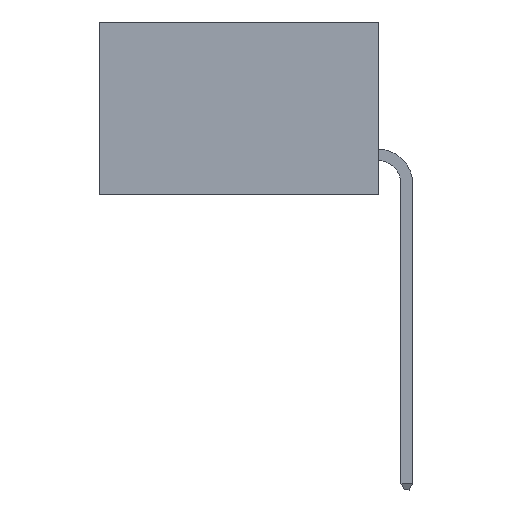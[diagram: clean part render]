
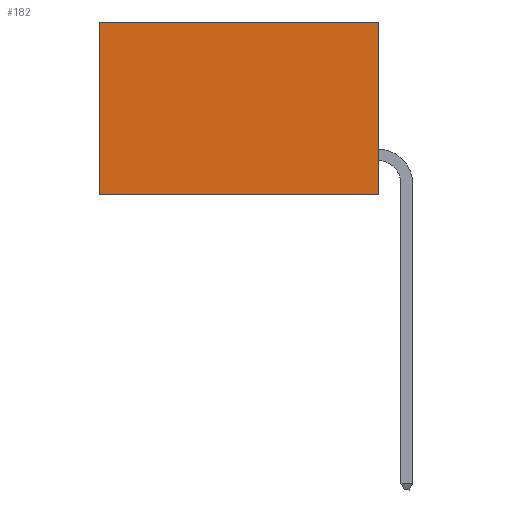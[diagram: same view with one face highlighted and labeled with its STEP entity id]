
A CAD part, left-side view. The second image highlights one B-rep face of the part: STEP entity #182.
In plain terms, the highlighted planar face has unit normal (-1, 0, 0).
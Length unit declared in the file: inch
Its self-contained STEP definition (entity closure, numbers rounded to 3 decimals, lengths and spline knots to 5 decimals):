
#182 = ADVANCED_FACE ( 'NONE', ( #12329 ), #8001, .F. ) ;
#435 = VERTEX_POINT ( 'NONE', #6025 ) ;
#619 = ORIENTED_EDGE ( 'NONE', *, *, #21745, .F. ) ;
#681 = CARTESIAN_POINT ( 'NONE',  ( 0.298, 0., 0. ) ) ;
#2143 = EDGE_LOOP ( 'NONE', ( #9115, #619, #16724, #24660 ) ) ;
#2857 = CARTESIAN_POINT ( 'NONE',  ( 0.298, 0.6, 0. ) ) ;
#3117 = EDGE_CURVE ( 'NONE', #23416, #435, #4865, .T. ) ;
#4064 = DIRECTION ( 'NONE',  ( 0., 1., 0. ) ) ;
#4679 = DIRECTION ( 'NONE',  ( 0., 0., -1. ) ) ;
#4865 = LINE ( 'NONE', #19541, #24991 ) ;
#5903 = LINE ( 'NONE', #12086, #15820 ) ;
#6025 = CARTESIAN_POINT ( 'NONE',  ( 0.298, 0., -0.37 ) ) ;
#6329 = CARTESIAN_POINT ( 'NONE',  ( 0.298, 0.6, -0.37 ) ) ;
#7411 = CARTESIAN_POINT ( 'NONE',  ( 0.298, 0., -0.37 ) ) ;
#7842 = DIRECTION ( 'NONE',  ( 0., 0., -1. ) ) ;
#8001 = PLANE ( 'NONE',  #11946 ) ;
#8317 = DIRECTION ( 'NONE',  ( 1., 0., 0. ) ) ;
#9115 = ORIENTED_EDGE ( 'NONE', *, *, #25028, .T. ) ;
#9404 = DIRECTION ( 'NONE',  ( 0., 1., 0. ) ) ;
#9970 = VERTEX_POINT ( 'NONE', #6329 ) ;
#10816 = VECTOR ( 'NONE', #18681, 39.37008 ) ;
#11425 = LINE ( 'NONE', #2857, #10816 ) ;
#11875 = LINE ( 'NONE', #7411, #21538 ) ;
#11946 = AXIS2_PLACEMENT_3D ( 'NONE', #18312, #8317, #4679 ) ;
#12086 = CARTESIAN_POINT ( 'NONE',  ( 0.298, 0., 0. ) ) ;
#12329 = FACE_OUTER_BOUND ( 'NONE', #2143, .T. ) ;
#15820 = VECTOR ( 'NONE', #4064, 39.37008 ) ;
#16724 = ORIENTED_EDGE ( 'NONE', *, *, #3117, .F. ) ;
#18312 = CARTESIAN_POINT ( 'NONE',  ( 0.298, 0., 0. ) ) ;
#18681 = DIRECTION ( 'NONE',  ( 0., 0., -1. ) ) ;
#19541 = CARTESIAN_POINT ( 'NONE',  ( 0.298, 0., 0. ) ) ;
#19553 = EDGE_CURVE ( 'NONE', #23416, #21923, #5903, .T. ) ;
#21538 = VECTOR ( 'NONE', #9404, 39.37008 ) ;
#21745 = EDGE_CURVE ( 'NONE', #435, #9970, #11875, .T. ) ;
#21923 = VERTEX_POINT ( 'NONE', #23444 ) ;
#23416 = VERTEX_POINT ( 'NONE', #681 ) ;
#23444 = CARTESIAN_POINT ( 'NONE',  ( 0.298, 0.6, 0. ) ) ;
#24660 = ORIENTED_EDGE ( 'NONE', *, *, #19553, .T. ) ;
#24991 = VECTOR ( 'NONE', #7842, 39.37008 ) ;
#25028 = EDGE_CURVE ( 'NONE', #21923, #9970, #11425, .T. ) ;
